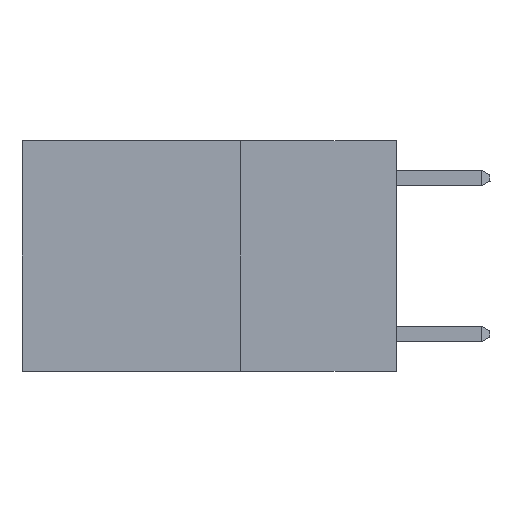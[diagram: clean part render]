
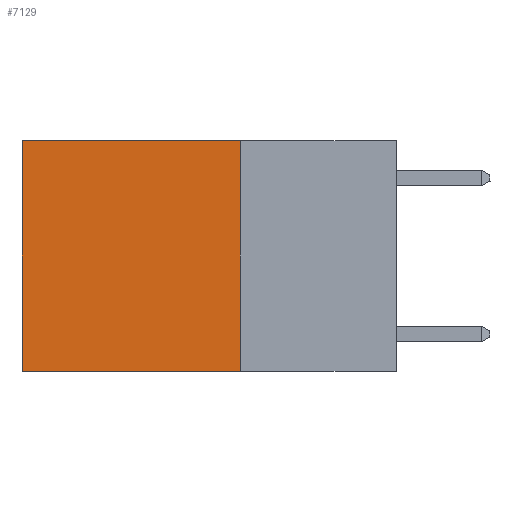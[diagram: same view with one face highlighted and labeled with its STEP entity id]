
A CAD part, left-side view. The second image highlights one B-rep face of the part: STEP entity #7129.
In plain terms, the highlighted planar face has unit normal (-1, 0, 0).
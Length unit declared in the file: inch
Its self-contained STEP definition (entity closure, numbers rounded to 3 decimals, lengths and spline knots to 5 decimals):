
#1013 = CARTESIAN_POINT ( 'NONE',  ( 0.2625, 0.6, 0. ) ) ;
#1405 = EDGE_CURVE ( 'NONE', #13547, #8087, #15448, .T. ) ;
#1589 = VECTOR ( 'NONE', #10025, 39.37008 ) ;
#2561 = ORIENTED_EDGE ( 'NONE', *, *, #1405, .F. ) ;
#2936 = CARTESIAN_POINT ( 'NONE',  ( 0.2625, 0.25, -0.37 ) ) ;
#3985 = DIRECTION ( 'NONE',  ( 0., 0., -1. ) ) ;
#4199 = VECTOR ( 'NONE', #3985, 39.37008 ) ;
#4320 = VECTOR ( 'NONE', #9104, 39.37008 ) ;
#4730 = EDGE_CURVE ( 'NONE', #13547, #20647, #18932, .T. ) ;
#6316 = CARTESIAN_POINT ( 'NONE',  ( 0.2625, 0.6, 0. ) ) ;
#6471 = ORIENTED_EDGE ( 'NONE', *, *, #4730, .T. ) ;
#7129 = ADVANCED_FACE ( 'NONE', ( #8467 ), #11562, .F. ) ;
#7626 = CARTESIAN_POINT ( 'NONE',  ( 0.2625, 0.25, 0. ) ) ;
#7850 = AXIS2_PLACEMENT_3D ( 'NONE', #14980, #22385, #15055 ) ;
#8087 = VERTEX_POINT ( 'NONE', #2936 ) ;
#8467 = FACE_OUTER_BOUND ( 'NONE', #21605, .T. ) ;
#9104 = DIRECTION ( 'NONE',  ( 0., 1., 0. ) ) ;
#9358 = LINE ( 'NONE', #6316, #13080 ) ;
#9394 = EDGE_CURVE ( 'NONE', #8087, #13660, #18452, .T. ) ;
#10025 = DIRECTION ( 'NONE',  ( 0., 1., 0. ) ) ;
#11562 = PLANE ( 'NONE',  #7850 ) ;
#11955 = EDGE_CURVE ( 'NONE', #20647, #13660, #9358, .T. ) ;
#13025 = ORIENTED_EDGE ( 'NONE', *, *, #9394, .F. ) ;
#13080 = VECTOR ( 'NONE', #15303, 39.37008 ) ;
#13547 = VERTEX_POINT ( 'NONE', #19273 ) ;
#13660 = VERTEX_POINT ( 'NONE', #17548 ) ;
#14980 = CARTESIAN_POINT ( 'NONE',  ( 0.2625, 0.25, 0. ) ) ;
#15055 = DIRECTION ( 'NONE',  ( 0., 0., -1. ) ) ;
#15303 = DIRECTION ( 'NONE',  ( 0., 0., -1. ) ) ;
#15448 = LINE ( 'NONE', #7626, #4199 ) ;
#15992 = CARTESIAN_POINT ( 'NONE',  ( 0.2625, 0.25, 0. ) ) ;
#17548 = CARTESIAN_POINT ( 'NONE',  ( 0.2625, 0.6, -0.37 ) ) ;
#18452 = LINE ( 'NONE', #19619, #4320 ) ;
#18932 = LINE ( 'NONE', #15992, #1589 ) ;
#19273 = CARTESIAN_POINT ( 'NONE',  ( 0.2625, 0.25, 0. ) ) ;
#19619 = CARTESIAN_POINT ( 'NONE',  ( 0.2625, 0.25, -0.37 ) ) ;
#20647 = VERTEX_POINT ( 'NONE', #1013 ) ;
#21605 = EDGE_LOOP ( 'NONE', ( #22030, #13025, #2561, #6471 ) ) ;
#22030 = ORIENTED_EDGE ( 'NONE', *, *, #11955, .T. ) ;
#22385 = DIRECTION ( 'NONE',  ( 1., 0., 0. ) ) ;
